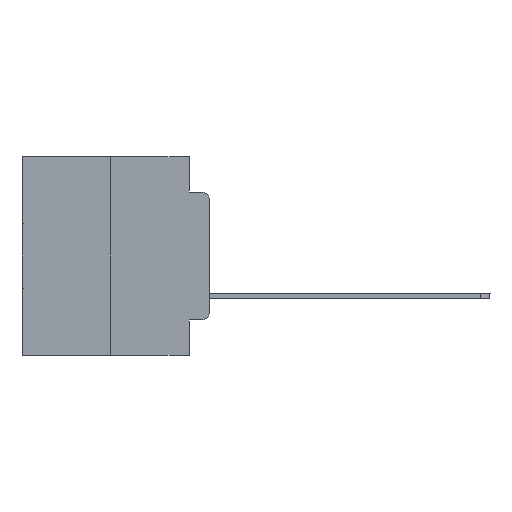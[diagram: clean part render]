
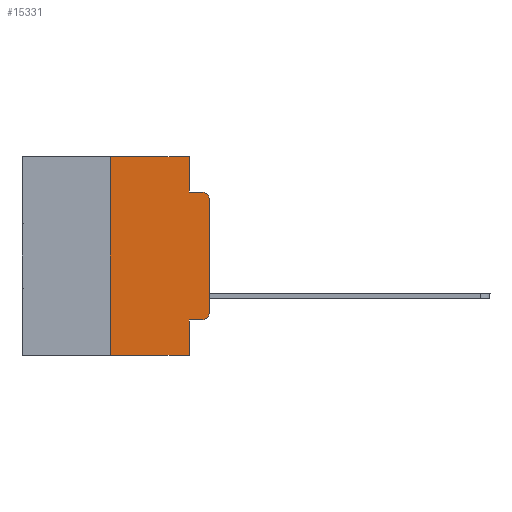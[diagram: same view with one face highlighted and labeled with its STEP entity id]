
A CAD part, left-side view. The second image highlights one B-rep face of the part: STEP entity #15331.
In plain terms, the highlighted planar face has unit normal (-1, 0, 0).
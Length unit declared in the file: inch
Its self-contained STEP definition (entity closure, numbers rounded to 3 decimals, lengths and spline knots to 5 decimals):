
#168 = CARTESIAN_POINT ( 'NONE',  ( 0., 0.051, -0.0885 ) ) ;
#239 = ORIENTED_EDGE ( 'NONE', *, *, #3084, .F. ) ;
#293 = ORIENTED_EDGE ( 'NONE', *, *, #9658, .F. ) ;
#483 = CARTESIAN_POINT ( 'NONE',  ( 0., 0.051, -0.4115 ) ) ;
#838 = ORIENTED_EDGE ( 'NONE', *, *, #5281, .T. ) ;
#2155 = EDGE_CURVE ( 'NONE', #19784, #19335, #24198, .T. ) ;
#2551 = CARTESIAN_POINT ( 'NONE',  ( 0., 0.473, -0.5 ) ) ;
#2596 = LINE ( 'NONE', #21407, #5628 ) ;
#3084 = EDGE_CURVE ( 'NONE', #24457, #29013, #19434, .T. ) ;
#3503 = DIRECTION ( 'NONE',  ( 0., -1., 0. ) ) ;
#4106 = ORIENTED_EDGE ( 'NONE', *, *, #2155, .T. ) ;
#4565 = VECTOR ( 'NONE', #7274, 39.37008 ) ;
#4864 = EDGE_CURVE ( 'NONE', #13129, #7654, #21099, .T. ) ;
#5281 = EDGE_CURVE ( 'NONE', #13129, #29013, #14287, .T. ) ;
#5628 = VECTOR ( 'NONE', #23119, 39.37008 ) ;
#6415 = LINE ( 'NONE', #9755, #24824 ) ;
#7191 = CARTESIAN_POINT ( 'NONE',  ( 0., 0.25, -0.5 ) ) ;
#7274 = DIRECTION ( 'NONE',  ( 0., -1., 0. ) ) ;
#7419 = EDGE_LOOP ( 'NONE', ( #29857, #10687, #26120, #293, #12447, #28557, #838, #239, #21686, #4106 ) ) ;
#7654 = VERTEX_POINT ( 'NONE', #27615 ) ;
#7801 = CARTESIAN_POINT ( 'NONE',  ( 0., 0.02, -0.1085 ) ) ;
#7965 = DIRECTION ( 'NONE',  ( 0., 0., -1. ) ) ;
#9658 = EDGE_CURVE ( 'NONE', #19585, #16801, #6415, .T. ) ;
#9755 = CARTESIAN_POINT ( 'NONE',  ( 0., 0.051, 0. ) ) ;
#10585 = EDGE_CURVE ( 'NONE', #14893, #29245, #11095, .T. ) ;
#10687 = ORIENTED_EDGE ( 'NONE', *, *, #10585, .T. ) ;
#10914 = CARTESIAN_POINT ( 'NONE',  ( 0., 0.051, 0. ) ) ;
#11085 = EDGE_CURVE ( 'NONE', #16801, #29245, #29285, .T. ) ;
#11095 = CIRCLE ( 'NONE', #23870, 0.02 ) ;
#11976 = DIRECTION ( 'NONE',  ( 0., -1., 0. ) ) ;
#12447 = ORIENTED_EDGE ( 'NONE', *, *, #29210, .F. ) ;
#12480 = DIRECTION ( 'NONE',  ( 1., 0., 0. ) ) ;
#13090 = CARTESIAN_POINT ( 'NONE',  ( 0., 0.473, 0. ) ) ;
#13129 = VERTEX_POINT ( 'NONE', #7191 ) ;
#14287 = LINE ( 'NONE', #2551, #26167 ) ;
#14407 = VECTOR ( 'NONE', #28212, 39.37008 ) ;
#14477 = CARTESIAN_POINT ( 'NONE',  ( 0., 0., -0.3915 ) ) ;
#14648 = CARTESIAN_POINT ( 'NONE',  ( 0., 0.051, 0. ) ) ;
#14792 = DIRECTION ( 'NONE',  ( 0., 0., -1. ) ) ;
#14893 = VERTEX_POINT ( 'NONE', #15286 ) ;
#14904 = DIRECTION ( 'NONE',  ( -1., 0., 0. ) ) ;
#14944 = VECTOR ( 'NONE', #28842, 39.37008 ) ;
#15098 = LINE ( 'NONE', #13090, #18669 ) ;
#15286 = CARTESIAN_POINT ( 'NONE',  ( 0., 0., -0.1085 ) ) ;
#15331 = ADVANCED_FACE ( 'NONE', ( #20819 ), #30231, .F. ) ;
#15563 = VECTOR ( 'NONE', #3503, 39.37008 ) ;
#15856 = AXIS2_PLACEMENT_3D ( 'NONE', #17436, #22201, #26825 ) ;
#16801 = VERTEX_POINT ( 'NONE', #30201 ) ;
#17436 = CARTESIAN_POINT ( 'NONE',  ( 0., 0.02, -0.3915 ) ) ;
#18669 = VECTOR ( 'NONE', #22487, 39.37008 ) ;
#18804 = CARTESIAN_POINT ( 'NONE',  ( 0., 0.25, 0. ) ) ;
#19273 = CARTESIAN_POINT ( 'NONE',  ( 0., 0.473, 0. ) ) ;
#19335 = VERTEX_POINT ( 'NONE', #14477 ) ;
#19434 = LINE ( 'NONE', #14648, #14944 ) ;
#19585 = VERTEX_POINT ( 'NONE', #10914 ) ;
#19784 = VERTEX_POINT ( 'NONE', #25702 ) ;
#19871 = CARTESIAN_POINT ( 'NONE',  ( 0., 0.02, -0.0885 ) ) ;
#20819 = FACE_OUTER_BOUND ( 'NONE', #7419, .T. ) ;
#21099 = LINE ( 'NONE', #18804, #14407 ) ;
#21407 = CARTESIAN_POINT ( 'NONE',  ( 0., 0., 0. ) ) ;
#21686 = ORIENTED_EDGE ( 'NONE', *, *, #21830, .T. ) ;
#21830 = EDGE_CURVE ( 'NONE', #24457, #19784, #28416, .T. ) ;
#22201 = DIRECTION ( 'NONE',  ( -1., 0., 0. ) ) ;
#22487 = DIRECTION ( 'NONE',  ( 0., -1., 0. ) ) ;
#23119 = DIRECTION ( 'NONE',  ( 0., 0., 1. ) ) ;
#23617 = CARTESIAN_POINT ( 'NONE',  ( 0., 0.051, -0.4115 ) ) ;
#23870 = AXIS2_PLACEMENT_3D ( 'NONE', #7801, #14904, #7965 ) ;
#24198 = CIRCLE ( 'NONE', #15856, 0.02 ) ;
#24457 = VERTEX_POINT ( 'NONE', #483 ) ;
#24824 = VECTOR ( 'NONE', #30170, 39.37008 ) ;
#25162 = EDGE_CURVE ( 'NONE', #19335, #14893, #2596, .T. ) ;
#25522 = AXIS2_PLACEMENT_3D ( 'NONE', #19273, #12480, #14792 ) ;
#25702 = CARTESIAN_POINT ( 'NONE',  ( 0., 0.02, -0.4115 ) ) ;
#26120 = ORIENTED_EDGE ( 'NONE', *, *, #11085, .F. ) ;
#26167 = VECTOR ( 'NONE', #11976, 39.37008 ) ;
#26825 = DIRECTION ( 'NONE',  ( 0., 0., -1. ) ) ;
#27615 = CARTESIAN_POINT ( 'NONE',  ( 0., 0.25, 0. ) ) ;
#28212 = DIRECTION ( 'NONE',  ( 0., 0., 1. ) ) ;
#28416 = LINE ( 'NONE', #23617, #4565 ) ;
#28557 = ORIENTED_EDGE ( 'NONE', *, *, #4864, .F. ) ;
#28842 = DIRECTION ( 'NONE',  ( 0., 0., -1. ) ) ;
#28983 = CARTESIAN_POINT ( 'NONE',  ( 0., 0.051, -0.5 ) ) ;
#29013 = VERTEX_POINT ( 'NONE', #28983 ) ;
#29210 = EDGE_CURVE ( 'NONE', #7654, #19585, #15098, .T. ) ;
#29245 = VERTEX_POINT ( 'NONE', #19871 ) ;
#29285 = LINE ( 'NONE', #168, #15563 ) ;
#29857 = ORIENTED_EDGE ( 'NONE', *, *, #25162, .T. ) ;
#30170 = DIRECTION ( 'NONE',  ( 0., 0., -1. ) ) ;
#30201 = CARTESIAN_POINT ( 'NONE',  ( 0., 0.051, -0.0885 ) ) ;
#30231 = PLANE ( 'NONE',  #25522 ) ;
